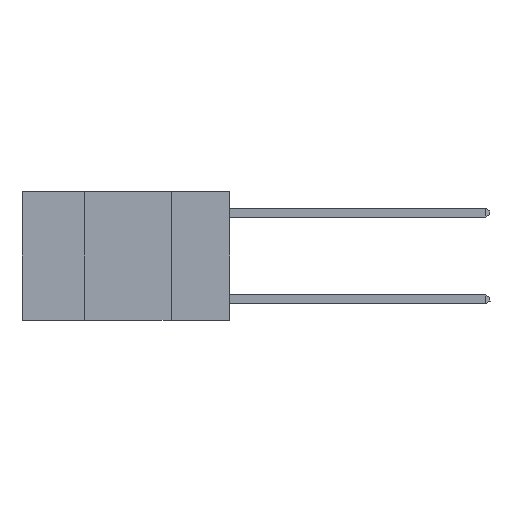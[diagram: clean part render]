
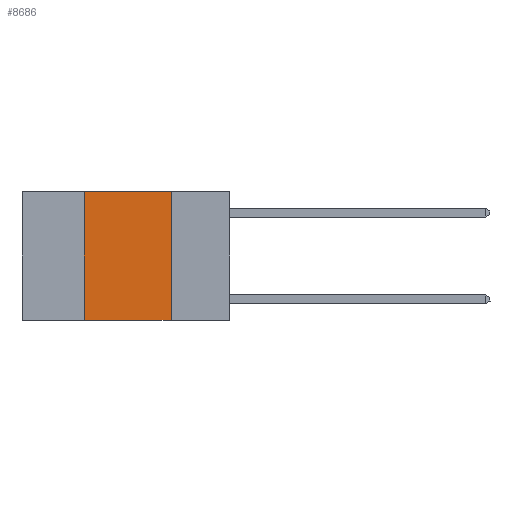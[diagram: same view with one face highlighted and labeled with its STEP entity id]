
A CAD part, left-side view. The second image highlights one B-rep face of the part: STEP entity #8686.
In plain terms, the highlighted planar face has unit normal (-1, 0, 0).
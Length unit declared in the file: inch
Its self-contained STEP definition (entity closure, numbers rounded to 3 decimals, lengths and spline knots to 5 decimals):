
#875 = CARTESIAN_POINT ( 'NONE',  ( 0., 0.6, 0. ) ) ;
#1505 = VECTOR ( 'NONE', #12443, 39.37008 ) ;
#1523 = CARTESIAN_POINT ( 'NONE',  ( 0., 0.17, -0.37 ) ) ;
#2287 = AXIS2_PLACEMENT_3D ( 'NONE', #21188, #16109, #6103 ) ;
#2385 = CARTESIAN_POINT ( 'NONE',  ( 0., 0.17, 0. ) ) ;
#2491 = ORIENTED_EDGE ( 'NONE', *, *, #5728, .F. ) ;
#3016 = ORIENTED_EDGE ( 'NONE', *, *, #4571, .T. ) ;
#4338 = CARTESIAN_POINT ( 'NONE',  ( 0., 0.42, 0. ) ) ;
#4374 = PLANE ( 'NONE',  #2287 ) ;
#4571 = EDGE_CURVE ( 'NONE', #15241, #16587, #14229, .T. ) ;
#5292 = VECTOR ( 'NONE', #16032, 39.37008 ) ;
#5728 = EDGE_CURVE ( 'NONE', #15241, #17021, #6585, .T. ) ;
#6048 = LINE ( 'NONE', #2385, #1505 ) ;
#6068 = FACE_OUTER_BOUND ( 'NONE', #6790, .T. ) ;
#6070 = DIRECTION ( 'NONE',  ( 0., 0., 1. ) ) ;
#6103 = DIRECTION ( 'NONE',  ( 0., 0., -1. ) ) ;
#6585 = LINE ( 'NONE', #4338, #18951 ) ;
#6790 = EDGE_LOOP ( 'NONE', ( #10924, #19894, #2491, #3016 ) ) ;
#8686 = ADVANCED_FACE ( 'NONE', ( #6068 ), #4374, .F. ) ;
#9139 = EDGE_CURVE ( 'NONE', #10520, #16587, #6048, .T. ) ;
#10520 = VERTEX_POINT ( 'NONE', #15897 ) ;
#10924 = ORIENTED_EDGE ( 'NONE', *, *, #9139, .F. ) ;
#11006 = CARTESIAN_POINT ( 'NONE',  ( 0., 0.6, -0.37 ) ) ;
#12443 = DIRECTION ( 'NONE',  ( 0., 0., -1. ) ) ;
#14051 = LINE ( 'NONE', #875, #18018 ) ;
#14229 = LINE ( 'NONE', #11006, #5292 ) ;
#14325 = CARTESIAN_POINT ( 'NONE',  ( 0., 0.42, 0. ) ) ;
#14467 = CARTESIAN_POINT ( 'NONE',  ( 0., 0.42, -0.37 ) ) ;
#15241 = VERTEX_POINT ( 'NONE', #14467 ) ;
#15897 = CARTESIAN_POINT ( 'NONE',  ( 0., 0.17, 0. ) ) ;
#16032 = DIRECTION ( 'NONE',  ( 0., -1., 0. ) ) ;
#16034 = DIRECTION ( 'NONE',  ( 0., -1., 0. ) ) ;
#16109 = DIRECTION ( 'NONE',  ( 1., 0., 0. ) ) ;
#16587 = VERTEX_POINT ( 'NONE', #1523 ) ;
#17021 = VERTEX_POINT ( 'NONE', #14325 ) ;
#18018 = VECTOR ( 'NONE', #16034, 39.37008 ) ;
#18951 = VECTOR ( 'NONE', #6070, 39.37008 ) ;
#19894 = ORIENTED_EDGE ( 'NONE', *, *, #21820, .F. ) ;
#21188 = CARTESIAN_POINT ( 'NONE',  ( 0., 0.6, 0. ) ) ;
#21820 = EDGE_CURVE ( 'NONE', #17021, #10520, #14051, .T. ) ;
